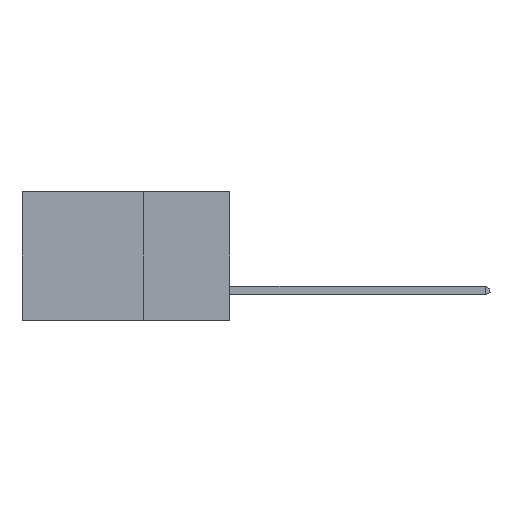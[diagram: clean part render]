
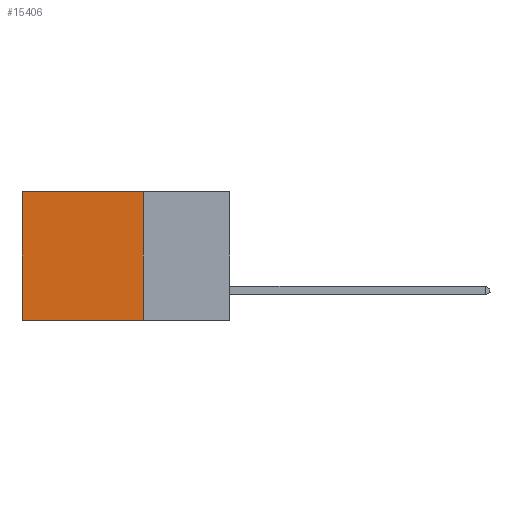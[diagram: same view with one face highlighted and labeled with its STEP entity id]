
A CAD part, left-side view. The second image highlights one B-rep face of the part: STEP entity #15406.
In plain terms, the highlighted planar face has unit normal (-1, 0, 0).
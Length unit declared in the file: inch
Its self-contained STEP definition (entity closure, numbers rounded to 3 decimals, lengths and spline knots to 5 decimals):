
#401 = VECTOR ( 'NONE', #1099, 39.37008 ) ;
#1099 = DIRECTION ( 'NONE',  ( 0., 1., 0. ) ) ;
#1338 = DIRECTION ( 'NONE',  ( 0., 0., -1. ) ) ;
#1846 = CARTESIAN_POINT ( 'NONE',  ( 0.298, 0.6, 0. ) ) ;
#2351 = EDGE_CURVE ( 'NONE', #15708, #22931, #28219, .T. ) ;
#3036 = ORIENTED_EDGE ( 'NONE', *, *, #18908, .F. ) ;
#3492 = FACE_OUTER_BOUND ( 'NONE', #23975, .T. ) ;
#3493 = VECTOR ( 'NONE', #17536, 39.37008 ) ;
#3824 = LINE ( 'NONE', #1846, #3493 ) ;
#4261 = PLANE ( 'NONE',  #5055 ) ;
#4404 = VERTEX_POINT ( 'NONE', #23163 ) ;
#5055 = AXIS2_PLACEMENT_3D ( 'NONE', #26803, #20305, #17916 ) ;
#5534 = VERTEX_POINT ( 'NONE', #5931 ) ;
#5653 = LINE ( 'NONE', #12402, #25394 ) ;
#5931 = CARTESIAN_POINT ( 'NONE',  ( 0.298, 0.6, -0.37 ) ) ;
#7639 = CARTESIAN_POINT ( 'NONE',  ( 0.298, 0.25, 0. ) ) ;
#8985 = CARTESIAN_POINT ( 'NONE',  ( 0.298, 0.6, 0. ) ) ;
#10234 = DIRECTION ( 'NONE',  ( 0., 1., 0. ) ) ;
#12402 = CARTESIAN_POINT ( 'NONE',  ( 0.298, 0.25, 0. ) ) ;
#12445 = CARTESIAN_POINT ( 'NONE',  ( 0.298, 0.25, 0. ) ) ;
#14371 = CARTESIAN_POINT ( 'NONE',  ( 0.298, 0.25, -0.37 ) ) ;
#15311 = ORIENTED_EDGE ( 'NONE', *, *, #28279, .T. ) ;
#15406 = ADVANCED_FACE ( 'NONE', ( #3492 ), #4261, .F. ) ;
#15519 = VECTOR ( 'NONE', #10234, 39.37008 ) ;
#15708 = VERTEX_POINT ( 'NONE', #7639 ) ;
#15722 = ORIENTED_EDGE ( 'NONE', *, *, #18996, .F. ) ;
#17536 = DIRECTION ( 'NONE',  ( 0., 0., -1. ) ) ;
#17916 = DIRECTION ( 'NONE',  ( 0., 0., -1. ) ) ;
#18908 = EDGE_CURVE ( 'NONE', #4404, #5534, #27565, .T. ) ;
#18996 = EDGE_CURVE ( 'NONE', #15708, #4404, #5653, .T. ) ;
#20305 = DIRECTION ( 'NONE',  ( 1., 0., 0. ) ) ;
#22931 = VERTEX_POINT ( 'NONE', #8985 ) ;
#23163 = CARTESIAN_POINT ( 'NONE',  ( 0.298, 0.25, -0.37 ) ) ;
#23467 = ORIENTED_EDGE ( 'NONE', *, *, #2351, .T. ) ;
#23975 = EDGE_LOOP ( 'NONE', ( #15311, #3036, #15722, #23467 ) ) ;
#25394 = VECTOR ( 'NONE', #1338, 39.37008 ) ;
#26803 = CARTESIAN_POINT ( 'NONE',  ( 0.298, 0.25, 0. ) ) ;
#27565 = LINE ( 'NONE', #14371, #15519 ) ;
#28219 = LINE ( 'NONE', #12445, #401 ) ;
#28279 = EDGE_CURVE ( 'NONE', #22931, #5534, #3824, .T. ) ;
